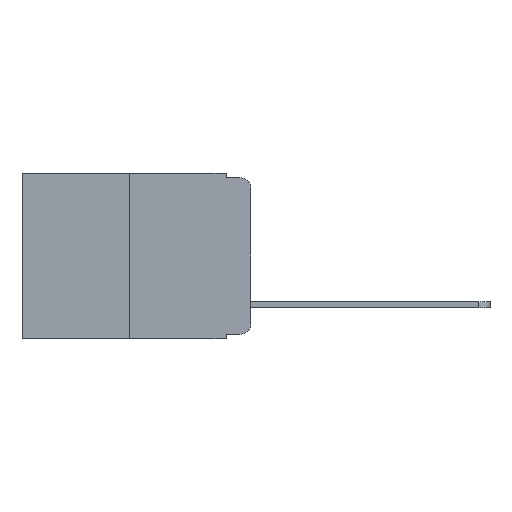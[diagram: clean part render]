
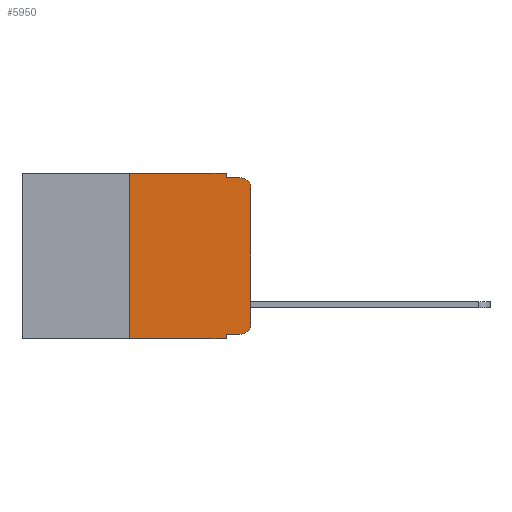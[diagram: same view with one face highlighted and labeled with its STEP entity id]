
A CAD part, left-side view. The second image highlights one B-rep face of the part: STEP entity #5950.
In plain terms, the highlighted planar face has unit normal (-1, 0, 0).
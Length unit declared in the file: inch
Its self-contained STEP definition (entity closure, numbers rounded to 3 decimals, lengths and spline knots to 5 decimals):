
#249 = EDGE_CURVE ( 'NONE', #7862, #10811, #1818, .T. ) ;
#494 = DIRECTION ( 'NONE',  ( 0., 0., -1. ) ) ;
#589 = CARTESIAN_POINT ( 'NONE',  ( 0., 0.473, 0. ) ) ;
#650 = VERTEX_POINT ( 'NONE', #7716 ) ;
#1061 = VECTOR ( 'NONE', #10298, 39.37008 ) ;
#1074 = VERTEX_POINT ( 'NONE', #4990 ) ;
#1209 = EDGE_CURVE ( 'NONE', #7862, #2798, #9148, .T. ) ;
#1818 = LINE ( 'NONE', #13256, #7355 ) ;
#2130 = LINE ( 'NONE', #9324, #4860 ) ;
#2524 = DIRECTION ( 'NONE',  ( 0., -1., 0. ) ) ;
#2656 = VECTOR ( 'NONE', #11184, 39.37008 ) ;
#2798 = VERTEX_POINT ( 'NONE', #9833 ) ;
#2890 = EDGE_CURVE ( 'NONE', #11415, #650, #11334, .T. ) ;
#2914 = EDGE_CURVE ( 'NONE', #11662, #9896, #10434, .T. ) ;
#2926 = CARTESIAN_POINT ( 'NONE',  ( 0., 0.051, 0. ) ) ;
#2937 = EDGE_CURVE ( 'NONE', #650, #3362, #2130, .T. ) ;
#2939 = CARTESIAN_POINT ( 'NONE',  ( 0., 0.02, -0.313 ) ) ;
#2947 = CARTESIAN_POINT ( 'NONE',  ( 0., 0.02, -0.333 ) ) ;
#2990 = CARTESIAN_POINT ( 'NONE',  ( 0., 0., 0. ) ) ;
#3362 = VERTEX_POINT ( 'NONE', #11178 ) ;
#4084 = DIRECTION ( 'NONE',  ( -1., 0., 0. ) ) ;
#4136 = DIRECTION ( 'NONE',  ( 0., 0., -1. ) ) ;
#4666 = LINE ( 'NONE', #589, #1061 ) ;
#4860 = VECTOR ( 'NONE', #12840, 39.37008 ) ;
#4990 = CARTESIAN_POINT ( 'NONE',  ( 0., 0., -0.313 ) ) ;
#5220 = VECTOR ( 'NONE', #8374, 39.37008 ) ;
#5252 = VERTEX_POINT ( 'NONE', #8525 ) ;
#5372 = ORIENTED_EDGE ( 'NONE', *, *, #8152, .T. ) ;
#5873 = VECTOR ( 'NONE', #2524, 39.37008 ) ;
#5950 = ADVANCED_FACE ( 'NONE', ( #10079 ), #8362, .F. ) ;
#6082 = ORIENTED_EDGE ( 'NONE', *, *, #8091, .T. ) ;
#6369 = CIRCLE ( 'NONE', #7813, 0.02 ) ;
#6711 = CARTESIAN_POINT ( 'NONE',  ( 0., 0.25, -0.343 ) ) ;
#6851 = CARTESIAN_POINT ( 'NONE',  ( 0., 0.051, -0.333 ) ) ;
#7254 = DIRECTION ( 'NONE',  ( 0., 0., -1. ) ) ;
#7301 = CARTESIAN_POINT ( 'NONE',  ( 0., 0.051, 0. ) ) ;
#7355 = VECTOR ( 'NONE', #8407, 39.37008 ) ;
#7401 = DIRECTION ( 'NONE',  ( 1., 0., 0. ) ) ;
#7705 = EDGE_LOOP ( 'NONE', ( #5372, #6082, #9591, #10880, #11337, #12057, #12792, #11224, #10693, #10951 ) ) ;
#7716 = CARTESIAN_POINT ( 'NONE',  ( 0., 0.051, -0.01 ) ) ;
#7790 = AXIS2_PLACEMENT_3D ( 'NONE', #2939, #10192, #4136 ) ;
#7813 = AXIS2_PLACEMENT_3D ( 'NONE', #10159, #4084, #11102 ) ;
#7862 = VERTEX_POINT ( 'NONE', #6851 ) ;
#7975 = CARTESIAN_POINT ( 'NONE',  ( 0., 0.473, -0.343 ) ) ;
#8091 = EDGE_CURVE ( 'NONE', #5252, #3362, #6369, .T. ) ;
#8118 = EDGE_CURVE ( 'NONE', #10811, #1074, #11193, .T. ) ;
#8152 = EDGE_CURVE ( 'NONE', #1074, #5252, #10899, .T. ) ;
#8362 = PLANE ( 'NONE',  #12540 ) ;
#8374 = DIRECTION ( 'NONE',  ( 0., 0., 1. ) ) ;
#8407 = DIRECTION ( 'NONE',  ( 0., -1., 0. ) ) ;
#8525 = CARTESIAN_POINT ( 'NONE',  ( 0., 0., -0.03 ) ) ;
#8635 = EDGE_CURVE ( 'NONE', #11662, #2798, #10721, .T. ) ;
#9148 = LINE ( 'NONE', #7301, #9462 ) ;
#9324 = CARTESIAN_POINT ( 'NONE',  ( 0., 0.051, -0.01 ) ) ;
#9462 = VECTOR ( 'NONE', #7254, 39.37008 ) ;
#9591 = ORIENTED_EDGE ( 'NONE', *, *, #2937, .F. ) ;
#9749 = EDGE_CURVE ( 'NONE', #9896, #11415, #4666, .T. ) ;
#9833 = CARTESIAN_POINT ( 'NONE',  ( 0., 0.051, -0.343 ) ) ;
#9896 = VERTEX_POINT ( 'NONE', #12398 ) ;
#10079 = FACE_OUTER_BOUND ( 'NONE', #7705, .T. ) ;
#10159 = CARTESIAN_POINT ( 'NONE',  ( 0., 0.02, -0.03 ) ) ;
#10192 = DIRECTION ( 'NONE',  ( -1., 0., 0. ) ) ;
#10298 = DIRECTION ( 'NONE',  ( 0., -1., 0. ) ) ;
#10434 = LINE ( 'NONE', #12643, #5220 ) ;
#10693 = ORIENTED_EDGE ( 'NONE', *, *, #249, .T. ) ;
#10721 = LINE ( 'NONE', #7975, #5873 ) ;
#10726 = VECTOR ( 'NONE', #11348, 39.37008 ) ;
#10811 = VERTEX_POINT ( 'NONE', #2947 ) ;
#10880 = ORIENTED_EDGE ( 'NONE', *, *, #2890, .F. ) ;
#10899 = LINE ( 'NONE', #2990, #2656 ) ;
#10951 = ORIENTED_EDGE ( 'NONE', *, *, #8118, .T. ) ;
#11102 = DIRECTION ( 'NONE',  ( 0., 0., -1. ) ) ;
#11178 = CARTESIAN_POINT ( 'NONE',  ( 0., 0.02, -0.01 ) ) ;
#11184 = DIRECTION ( 'NONE',  ( 0., 0., 1. ) ) ;
#11193 = CIRCLE ( 'NONE', #7790, 0.02 ) ;
#11224 = ORIENTED_EDGE ( 'NONE', *, *, #1209, .F. ) ;
#11334 = LINE ( 'NONE', #12883, #10726 ) ;
#11337 = ORIENTED_EDGE ( 'NONE', *, *, #9749, .F. ) ;
#11348 = DIRECTION ( 'NONE',  ( 0., 0., -1. ) ) ;
#11415 = VERTEX_POINT ( 'NONE', #2926 ) ;
#11662 = VERTEX_POINT ( 'NONE', #6711 ) ;
#12057 = ORIENTED_EDGE ( 'NONE', *, *, #2914, .F. ) ;
#12398 = CARTESIAN_POINT ( 'NONE',  ( 0., 0.25, 0. ) ) ;
#12540 = AXIS2_PLACEMENT_3D ( 'NONE', #12969, #7401, #494 ) ;
#12643 = CARTESIAN_POINT ( 'NONE',  ( 0., 0.25, 0. ) ) ;
#12792 = ORIENTED_EDGE ( 'NONE', *, *, #8635, .T. ) ;
#12840 = DIRECTION ( 'NONE',  ( 0., -1., 0. ) ) ;
#12883 = CARTESIAN_POINT ( 'NONE',  ( 0., 0.051, 0. ) ) ;
#12969 = CARTESIAN_POINT ( 'NONE',  ( 0., 0.473, 0. ) ) ;
#13256 = CARTESIAN_POINT ( 'NONE',  ( 0., 0.051, -0.333 ) ) ;
